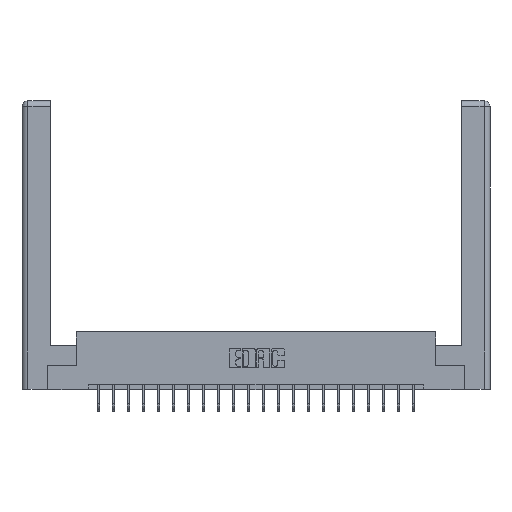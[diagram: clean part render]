
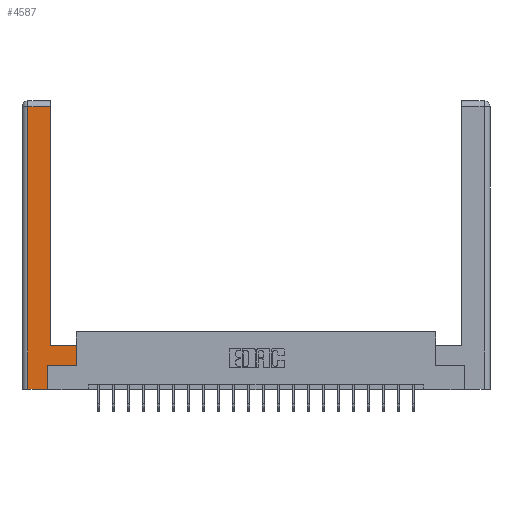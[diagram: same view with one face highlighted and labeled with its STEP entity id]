
A CAD part, top view. The second image highlights one B-rep face of the part: STEP entity #4587.
In plain terms, the highlighted planar face has unit normal (0, 0, 1).
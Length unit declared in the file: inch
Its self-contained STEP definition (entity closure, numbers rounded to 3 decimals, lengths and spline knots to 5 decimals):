
#618 = FACE_OUTER_BOUND ( 'NONE', #11299, .T. ) ;
#859 = CARTESIAN_POINT ( 'NONE',  ( 0.265, 0.245, 0. ) ) ;
#1006 = VECTOR ( 'NONE', #10078, 39.37008 ) ;
#1122 = CARTESIAN_POINT ( 'NONE',  ( 0.265, 0., 0. ) ) ;
#1333 = LINE ( 'NONE', #1122, #1006 ) ;
#1671 = ORIENTED_EDGE ( 'NONE', *, *, #20209, .T. ) ;
#1977 = VECTOR ( 'NONE', #17830, 39.37008 ) ;
#2250 = LINE ( 'NONE', #9870, #17350 ) ;
#3059 = CARTESIAN_POINT ( 'NONE',  ( 0.295, 2.94, 0. ) ) ;
#3698 = EDGE_CURVE ( 'NONE', #17427, #11896, #4440, .T. ) ;
#4065 = DIRECTION ( 'NONE',  ( -1., 0., 0. ) ) ;
#4440 = LINE ( 'NONE', #13555, #10534 ) ;
#4587 = ADVANCED_FACE ( 'NONE', ( #618 ), #15799, .F. ) ;
#4903 = VECTOR ( 'NONE', #4065, 39.37008 ) ;
#5456 = VECTOR ( 'NONE', #12503, 39.37008 ) ;
#6415 = VERTEX_POINT ( 'NONE', #14544 ) ;
#6479 = DIRECTION ( 'NONE',  ( -1., 0., 0. ) ) ;
#7211 = EDGE_CURVE ( 'NONE', #20293, #17427, #13852, .T. ) ;
#7493 = EDGE_CURVE ( 'NONE', #11896, #14873, #9179, .T. ) ;
#9179 = LINE ( 'NONE', #14585, #5456 ) ;
#9870 = CARTESIAN_POINT ( 'NONE',  ( 0.565, 0.45, 0. ) ) ;
#10045 = DIRECTION ( 'NONE',  ( 1., 0., 0. ) ) ;
#10078 = DIRECTION ( 'NONE',  ( 1., 0., 0. ) ) ;
#10129 = DIRECTION ( 'NONE',  ( 0., 0., -1. ) ) ;
#10183 = VECTOR ( 'NONE', #10045, 39.37008 ) ;
#10353 = EDGE_CURVE ( 'NONE', #19521, #15271, #15774, .T. ) ;
#10534 = VECTOR ( 'NONE', #15170, 39.37008 ) ;
#10908 = ORIENTED_EDGE ( 'NONE', *, *, #7493, .T. ) ;
#11055 = LINE ( 'NONE', #19565, #10183 ) ;
#11259 = ORIENTED_EDGE ( 'NONE', *, *, #12861, .T. ) ;
#11299 = EDGE_LOOP ( 'NONE', ( #21538, #10908, #1671, #11259, #21701, #19950, #19424, #13411 ) ) ;
#11418 = VECTOR ( 'NONE', #23458, 39.37008 ) ;
#11479 = CARTESIAN_POINT ( 'NONE',  ( 0.0615, 2.94, 0. ) ) ;
#11725 = DIRECTION ( 'NONE',  ( 0., 1., 0. ) ) ;
#11896 = VERTEX_POINT ( 'NONE', #3059 ) ;
#12503 = DIRECTION ( 'NONE',  ( -1., 0., 0. ) ) ;
#12861 = EDGE_CURVE ( 'NONE', #6415, #19521, #1333, .T. ) ;
#13411 = ORIENTED_EDGE ( 'NONE', *, *, #7211, .T. ) ;
#13555 = CARTESIAN_POINT ( 'NONE',  ( 0.295, 3., 0. ) ) ;
#13852 = LINE ( 'NONE', #15159, #4903 ) ;
#14343 = CARTESIAN_POINT ( 'NONE',  ( 0.265, 0.245, 0. ) ) ;
#14544 = CARTESIAN_POINT ( 'NONE',  ( 0.0615, 0., 0. ) ) ;
#14585 = CARTESIAN_POINT ( 'NONE',  ( 0.0615, 2.94, 0. ) ) ;
#14873 = VERTEX_POINT ( 'NONE', #11479 ) ;
#15159 = CARTESIAN_POINT ( 'NONE',  ( 0.295, 0.45, 0. ) ) ;
#15170 = DIRECTION ( 'NONE',  ( 0., 1., 0. ) ) ;
#15271 = VERTEX_POINT ( 'NONE', #859 ) ;
#15363 = CARTESIAN_POINT ( 'NONE',  ( 0.265, 0., 0. ) ) ;
#15774 = LINE ( 'NONE', #14343, #11418 ) ;
#15799 = PLANE ( 'NONE',  #18457 ) ;
#17350 = VECTOR ( 'NONE', #11725, 39.37008 ) ;
#17427 = VERTEX_POINT ( 'NONE', #20527 ) ;
#17656 = CARTESIAN_POINT ( 'NONE',  ( 0.565, 0.245, 0. ) ) ;
#17830 = DIRECTION ( 'NONE',  ( 0., -1., 0. ) ) ;
#18457 = AXIS2_PLACEMENT_3D ( 'NONE', #19559, #10129, #6479 ) ;
#18576 = VERTEX_POINT ( 'NONE', #17656 ) ;
#19424 = ORIENTED_EDGE ( 'NONE', *, *, #23268, .T. ) ;
#19521 = VERTEX_POINT ( 'NONE', #15363 ) ;
#19559 = CARTESIAN_POINT ( 'NONE',  ( 0., 0., 0. ) ) ;
#19565 = CARTESIAN_POINT ( 'NONE',  ( 0.565, 0.245, 0. ) ) ;
#19950 = ORIENTED_EDGE ( 'NONE', *, *, #21446, .T. ) ;
#20209 = EDGE_CURVE ( 'NONE', #14873, #6415, #23496, .T. ) ;
#20293 = VERTEX_POINT ( 'NONE', #21496 ) ;
#20527 = CARTESIAN_POINT ( 'NONE',  ( 0.295, 0.45, 0. ) ) ;
#21446 = EDGE_CURVE ( 'NONE', #15271, #18576, #11055, .T. ) ;
#21496 = CARTESIAN_POINT ( 'NONE',  ( 0.565, 0.45, 0. ) ) ;
#21538 = ORIENTED_EDGE ( 'NONE', *, *, #3698, .T. ) ;
#21701 = ORIENTED_EDGE ( 'NONE', *, *, #10353, .T. ) ;
#23268 = EDGE_CURVE ( 'NONE', #18576, #20293, #2250, .T. ) ;
#23458 = DIRECTION ( 'NONE',  ( 0., 1., 0. ) ) ;
#23496 = LINE ( 'NONE', #23616, #1977 ) ;
#23616 = CARTESIAN_POINT ( 'NONE',  ( 0.0615, 0., 0. ) ) ;
